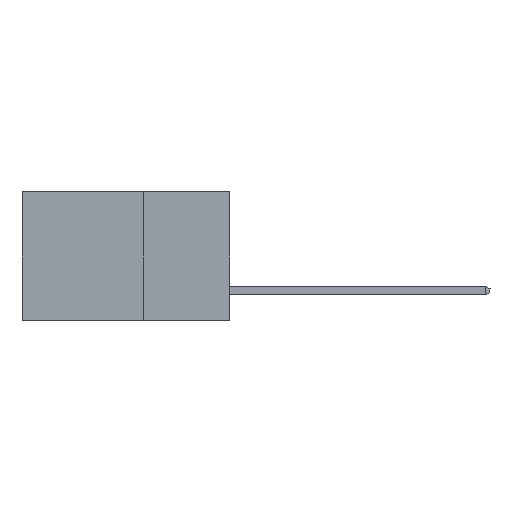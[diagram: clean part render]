
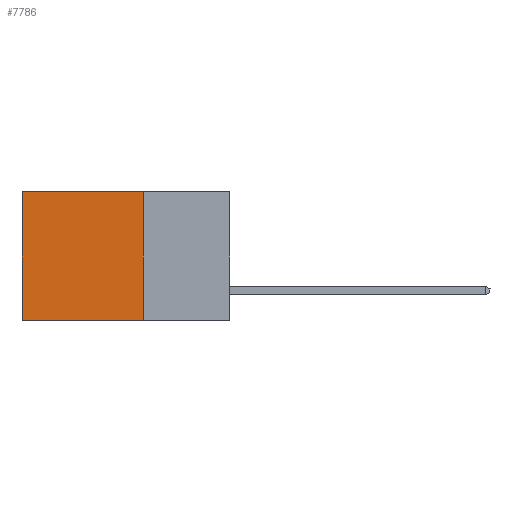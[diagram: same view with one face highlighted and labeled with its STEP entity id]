
A CAD part, left-side view. The second image highlights one B-rep face of the part: STEP entity #7786.
In plain terms, the highlighted planar face has unit normal (-1, 0, 0).
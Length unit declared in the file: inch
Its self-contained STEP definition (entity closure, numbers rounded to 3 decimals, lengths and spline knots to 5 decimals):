
#734 = AXIS2_PLACEMENT_3D ( 'NONE', #2867, #14228, #12876 ) ;
#1174 = LINE ( 'NONE', #13714, #7247 ) ;
#2083 = LINE ( 'NONE', #7301, #11019 ) ;
#2503 = CARTESIAN_POINT ( 'NONE',  ( 0.2615, 0.6, -0.37 ) ) ;
#2867 = CARTESIAN_POINT ( 'NONE',  ( 0.2615, 0.25, -0.37 ) ) ;
#3074 = ORIENTED_EDGE ( 'NONE', *, *, #5115, .T. ) ;
#3591 = EDGE_LOOP ( 'NONE', ( #3074, #7501, #10289, #12143 ) ) ;
#3830 = LINE ( 'NONE', #15056, #15097 ) ;
#4002 = PLANE ( 'NONE',  #734 ) ;
#4636 = VERTEX_POINT ( 'NONE', #2503 ) ;
#4942 = VECTOR ( 'NONE', #14520, 39.37008 ) ;
#5065 = VERTEX_POINT ( 'NONE', #7535 ) ;
#5115 = EDGE_CURVE ( 'NONE', #14324, #4636, #1174, .T. ) ;
#5529 = FACE_OUTER_BOUND ( 'NONE', #3591, .T. ) ;
#7052 = DIRECTION ( 'NONE',  ( 0., 1., 0. ) ) ;
#7247 = VECTOR ( 'NONE', #9893, 39.37008 ) ;
#7301 = CARTESIAN_POINT ( 'NONE',  ( 0.2615, 0.25, 0. ) ) ;
#7501 = ORIENTED_EDGE ( 'NONE', *, *, #9478, .F. ) ;
#7535 = CARTESIAN_POINT ( 'NONE',  ( 0.2615, 0.25, -0.37 ) ) ;
#7786 = ADVANCED_FACE ( 'NONE', ( #5529 ), #4002, .F. ) ;
#8352 = CARTESIAN_POINT ( 'NONE',  ( 0.2615, 0.25, 0. ) ) ;
#8365 = CARTESIAN_POINT ( 'NONE',  ( 0.2615, 0.6, 0. ) ) ;
#8800 = VERTEX_POINT ( 'NONE', #8352 ) ;
#8836 = EDGE_CURVE ( 'NONE', #8800, #5065, #10532, .T. ) ;
#9478 = EDGE_CURVE ( 'NONE', #5065, #4636, #3830, .T. ) ;
#9893 = DIRECTION ( 'NONE',  ( 0., 0., -1. ) ) ;
#10289 = ORIENTED_EDGE ( 'NONE', *, *, #8836, .F. ) ;
#10532 = LINE ( 'NONE', #10776, #4942 ) ;
#10776 = CARTESIAN_POINT ( 'NONE',  ( 0.2615, 0.25, -0.37 ) ) ;
#11019 = VECTOR ( 'NONE', #7052, 39.37008 ) ;
#11063 = DIRECTION ( 'NONE',  ( 0., 1., 0. ) ) ;
#11803 = EDGE_CURVE ( 'NONE', #8800, #14324, #2083, .T. ) ;
#12143 = ORIENTED_EDGE ( 'NONE', *, *, #11803, .T. ) ;
#12876 = DIRECTION ( 'NONE',  ( 0., 0., -1. ) ) ;
#13714 = CARTESIAN_POINT ( 'NONE',  ( 0.2615, 0.6, -0.37 ) ) ;
#14228 = DIRECTION ( 'NONE',  ( 1., 0., 0. ) ) ;
#14324 = VERTEX_POINT ( 'NONE', #8365 ) ;
#14520 = DIRECTION ( 'NONE',  ( 0., 0., -1. ) ) ;
#15056 = CARTESIAN_POINT ( 'NONE',  ( 0.2615, 0.25, -0.37 ) ) ;
#15097 = VECTOR ( 'NONE', #11063, 39.37008 ) ;
